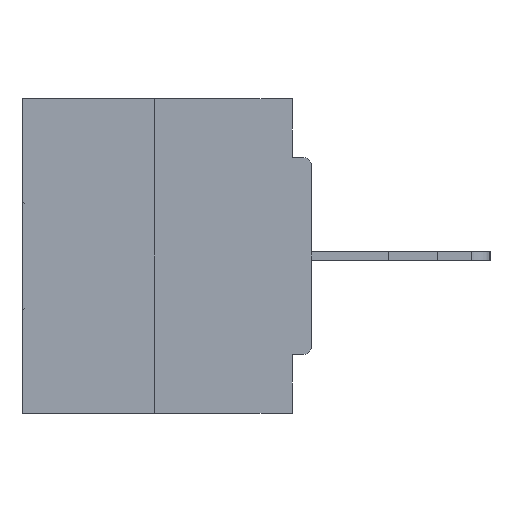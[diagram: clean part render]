
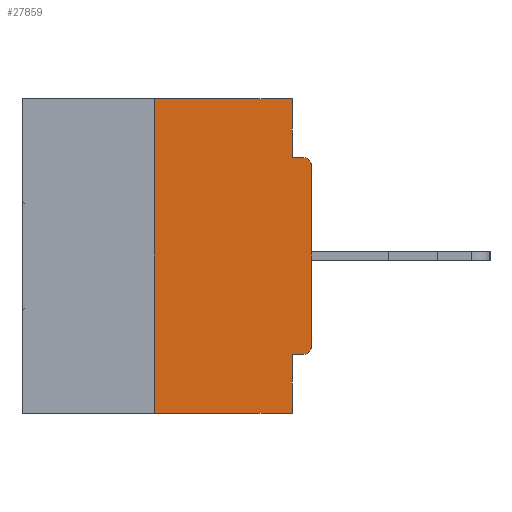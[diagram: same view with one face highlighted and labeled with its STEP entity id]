
A CAD part, left-side view. The second image highlights one B-rep face of the part: STEP entity #27859.
In plain terms, the highlighted planar face has unit normal (-1, 0, 0).
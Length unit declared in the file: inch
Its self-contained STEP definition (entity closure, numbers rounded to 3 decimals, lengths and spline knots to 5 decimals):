
#300 = CARTESIAN_POINT ( 'NONE',  ( 0., 0.25, 0. ) ) ;
#376 = DIRECTION ( 'NONE',  ( 1., 0., 0. ) ) ;
#925 = ORIENTED_EDGE ( 'NONE', *, *, #7403, .F. ) ;
#1100 = VERTEX_POINT ( 'NONE', #11333 ) ;
#1603 = CARTESIAN_POINT ( 'NONE',  ( 0., 0.031, -0.0935 ) ) ;
#1616 = ORIENTED_EDGE ( 'NONE', *, *, #18168, .T. ) ;
#1643 = CARTESIAN_POINT ( 'NONE',  ( 0., 0., -0.3915 ) ) ;
#1850 = VERTEX_POINT ( 'NONE', #12409 ) ;
#2142 = EDGE_CURVE ( 'NONE', #7339, #1850, #27449, .T. ) ;
#2178 = LINE ( 'NONE', #34245, #31923 ) ;
#2410 = DIRECTION ( 'NONE',  ( -1., 0., 0. ) ) ;
#2856 = DIRECTION ( 'NONE',  ( 0., 0., -1. ) ) ;
#3058 = LINE ( 'NONE', #27596, #22840 ) ;
#4389 = DIRECTION ( 'NONE',  ( 0., 0., -1. ) ) ;
#4956 = LINE ( 'NONE', #31576, #34652 ) ;
#4982 = EDGE_CURVE ( 'NONE', #14833, #23791, #3058, .T. ) ;
#5149 = ORIENTED_EDGE ( 'NONE', *, *, #2142, .T. ) ;
#5825 = PLANE ( 'NONE',  #7522 ) ;
#6276 = EDGE_LOOP ( 'NONE', ( #925, #12754, #5149, #15302, #12191, #18637, #1616, #7467, #32601, #11261 ) ) ;
#7339 = VERTEX_POINT ( 'NONE', #30484 ) ;
#7403 = EDGE_CURVE ( 'NONE', #35753, #14833, #17302, .T. ) ;
#7467 = ORIENTED_EDGE ( 'NONE', *, *, #9142, .T. ) ;
#7522 = AXIS2_PLACEMENT_3D ( 'NONE', #8737, #376, #26278 ) ;
#8126 = CARTESIAN_POINT ( 'NONE',  ( 0., 0., -0.0935 ) ) ;
#8302 = EDGE_CURVE ( 'NONE', #7339, #35753, #14968, .T. ) ;
#8493 = DIRECTION ( 'NONE',  ( 0., 1., 0. ) ) ;
#8665 = CARTESIAN_POINT ( 'NONE',  ( 0., 0.46, -0.5 ) ) ;
#8737 = CARTESIAN_POINT ( 'NONE',  ( 0., 0.46, 0. ) ) ;
#9142 = EDGE_CURVE ( 'NONE', #1100, #24432, #30234, .T. ) ;
#10214 = AXIS2_PLACEMENT_3D ( 'NONE', #28296, #2410, #28063 ) ;
#11261 = ORIENTED_EDGE ( 'NONE', *, *, #4982, .F. ) ;
#11333 = CARTESIAN_POINT ( 'NONE',  ( 0., 0., -0.1085 ) ) ;
#11828 = CARTESIAN_POINT ( 'NONE',  ( 0., 0.031, -0.4065 ) ) ;
#12191 = ORIENTED_EDGE ( 'NONE', *, *, #31594, .F. ) ;
#12409 = CARTESIAN_POINT ( 'NONE',  ( 0., 0.031, -0.5 ) ) ;
#12754 = ORIENTED_EDGE ( 'NONE', *, *, #8302, .F. ) ;
#13435 = DIRECTION ( 'NONE',  ( 0., 0., 1. ) ) ;
#13809 = VECTOR ( 'NONE', #25207, 39.37008 ) ;
#14007 = DIRECTION ( 'NONE',  ( 0., -1., 0. ) ) ;
#14833 = VERTEX_POINT ( 'NONE', #17785 ) ;
#14968 = LINE ( 'NONE', #27916, #19908 ) ;
#15302 = ORIENTED_EDGE ( 'NONE', *, *, #17071, .F. ) ;
#17071 = EDGE_CURVE ( 'NONE', #24878, #1850, #36736, .T. ) ;
#17302 = LINE ( 'NONE', #22017, #33036 ) ;
#17785 = CARTESIAN_POINT ( 'NONE',  ( 0., 0.031, 0. ) ) ;
#18168 = EDGE_CURVE ( 'NONE', #36396, #1100, #4956, .T. ) ;
#18573 = CARTESIAN_POINT ( 'NONE',  ( 0., 0.015, -0.4065 ) ) ;
#18637 = ORIENTED_EDGE ( 'NONE', *, *, #20352, .T. ) ;
#19908 = VECTOR ( 'NONE', #13435, 39.37008 ) ;
#20071 = DIRECTION ( 'NONE',  ( -1., 0., 0. ) ) ;
#20352 = EDGE_CURVE ( 'NONE', #32259, #36396, #27051, .T. ) ;
#21376 = CARTESIAN_POINT ( 'NONE',  ( 0., 0.015, -0.0935 ) ) ;
#21602 = CARTESIAN_POINT ( 'NONE',  ( 0., 0.031, -0.5 ) ) ;
#22017 = CARTESIAN_POINT ( 'NONE',  ( 0., 0.46, 0. ) ) ;
#22840 = VECTOR ( 'NONE', #30785, 39.37008 ) ;
#23791 = VERTEX_POINT ( 'NONE', #1603 ) ;
#24432 = VERTEX_POINT ( 'NONE', #21376 ) ;
#24878 = VERTEX_POINT ( 'NONE', #11828 ) ;
#25207 = DIRECTION ( 'NONE',  ( 0., -1., 0. ) ) ;
#26278 = DIRECTION ( 'NONE',  ( 0., 0., -1. ) ) ;
#26563 = VECTOR ( 'NONE', #14007, 39.37008 ) ;
#27051 = CIRCLE ( 'NONE', #10214, 0.015 ) ;
#27267 = EDGE_CURVE ( 'NONE', #23791, #24432, #30051, .T. ) ;
#27449 = LINE ( 'NONE', #8665, #26563 ) ;
#27596 = CARTESIAN_POINT ( 'NONE',  ( 0., 0.031, 0. ) ) ;
#27859 = ADVANCED_FACE ( 'NONE', ( #28625 ), #5825, .F. ) ;
#27916 = CARTESIAN_POINT ( 'NONE',  ( 0., 0.25, 0. ) ) ;
#28063 = DIRECTION ( 'NONE',  ( 0., 0., -1. ) ) ;
#28296 = CARTESIAN_POINT ( 'NONE',  ( 0., 0.015, -0.3915 ) ) ;
#28625 = FACE_OUTER_BOUND ( 'NONE', #6276, .T. ) ;
#30051 = LINE ( 'NONE', #8126, #13809 ) ;
#30234 = CIRCLE ( 'NONE', #31281, 0.015 ) ;
#30484 = CARTESIAN_POINT ( 'NONE',  ( 0., 0.25, -0.5 ) ) ;
#30785 = DIRECTION ( 'NONE',  ( 0., 0., -1. ) ) ;
#30925 = VECTOR ( 'NONE', #4389, 39.37008 ) ;
#31281 = AXIS2_PLACEMENT_3D ( 'NONE', #37312, #20071, #2856 ) ;
#31576 = CARTESIAN_POINT ( 'NONE',  ( 0., 0., 0. ) ) ;
#31594 = EDGE_CURVE ( 'NONE', #32259, #24878, #2178, .T. ) ;
#31923 = VECTOR ( 'NONE', #8493, 39.37008 ) ;
#32259 = VERTEX_POINT ( 'NONE', #18573 ) ;
#32601 = ORIENTED_EDGE ( 'NONE', *, *, #27267, .F. ) ;
#33036 = VECTOR ( 'NONE', #36731, 39.37008 ) ;
#34245 = CARTESIAN_POINT ( 'NONE',  ( 0., 0., -0.4065 ) ) ;
#34576 = DIRECTION ( 'NONE',  ( 0., 0., 1. ) ) ;
#34652 = VECTOR ( 'NONE', #34576, 39.37008 ) ;
#35753 = VERTEX_POINT ( 'NONE', #300 ) ;
#36396 = VERTEX_POINT ( 'NONE', #1643 ) ;
#36731 = DIRECTION ( 'NONE',  ( 0., -1., 0. ) ) ;
#36736 = LINE ( 'NONE', #21602, #30925 ) ;
#37312 = CARTESIAN_POINT ( 'NONE',  ( 0., 0.015, -0.1085 ) ) ;
